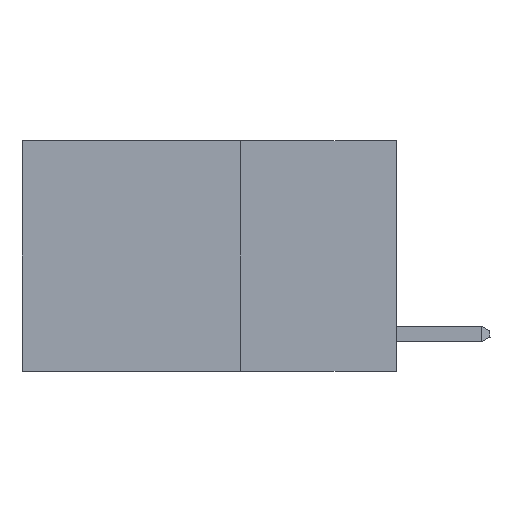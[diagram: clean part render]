
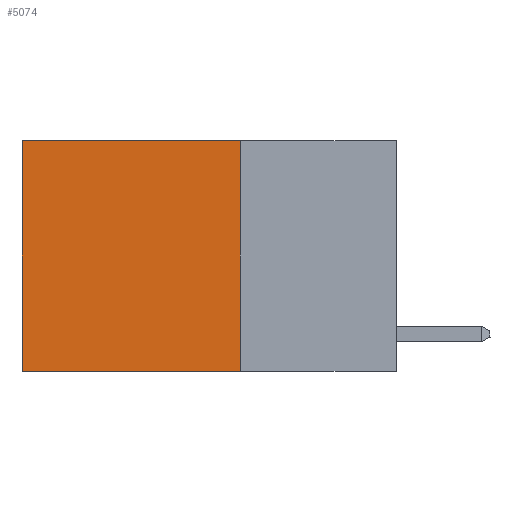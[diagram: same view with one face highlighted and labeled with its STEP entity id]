
A CAD part, left-side view. The second image highlights one B-rep face of the part: STEP entity #5074.
In plain terms, the highlighted planar face has unit normal (-1, 0, 0).
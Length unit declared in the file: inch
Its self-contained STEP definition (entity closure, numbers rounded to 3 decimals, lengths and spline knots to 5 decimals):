
#591 = LINE ( 'NONE', #10597, #12261 ) ;
#614 = VECTOR ( 'NONE', #5404, 39.37008 ) ;
#617 = CARTESIAN_POINT ( 'NONE',  ( 0.2625, 0.25, 0. ) ) ;
#834 = ORIENTED_EDGE ( 'NONE', *, *, #8151, .F. ) ;
#877 = CARTESIAN_POINT ( 'NONE',  ( 0.2625, 0.25, 0. ) ) ;
#1131 = DIRECTION ( 'NONE',  ( 0., 0., -1. ) ) ;
#1526 = VERTEX_POINT ( 'NONE', #4899 ) ;
#1620 = CARTESIAN_POINT ( 'NONE',  ( 0.2625, 0.6, 0. ) ) ;
#3361 = CARTESIAN_POINT ( 'NONE',  ( 0.2625, 0.25, 0. ) ) ;
#3754 = CARTESIAN_POINT ( 'NONE',  ( 0.2625, 0.6, -0.37 ) ) ;
#3759 = ORIENTED_EDGE ( 'NONE', *, *, #8839, .T. ) ;
#3960 = LINE ( 'NONE', #8099, #12637 ) ;
#4899 = CARTESIAN_POINT ( 'NONE',  ( 0.2625, 0.25, -0.37 ) ) ;
#5074 = ADVANCED_FACE ( 'NONE', ( #6721 ), #5600, .F. ) ;
#5404 = DIRECTION ( 'NONE',  ( 0., 1., 0. ) ) ;
#5600 = PLANE ( 'NONE',  #6029 ) ;
#6029 = AXIS2_PLACEMENT_3D ( 'NONE', #3361, #7900, #1131 ) ;
#6721 = FACE_OUTER_BOUND ( 'NONE', #7331, .T. ) ;
#7331 = EDGE_LOOP ( 'NONE', ( #3759, #9651, #834, #7700 ) ) ;
#7636 = DIRECTION ( 'NONE',  ( 0., 0., -1. ) ) ;
#7700 = ORIENTED_EDGE ( 'NONE', *, *, #9796, .T. ) ;
#7900 = DIRECTION ( 'NONE',  ( 1., 0., 0. ) ) ;
#8099 = CARTESIAN_POINT ( 'NONE',  ( 0.2625, 0.6, 0. ) ) ;
#8151 = EDGE_CURVE ( 'NONE', #13231, #1526, #8583, .T. ) ;
#8583 = LINE ( 'NONE', #877, #14257 ) ;
#8839 = EDGE_CURVE ( 'NONE', #14494, #13821, #3960, .T. ) ;
#9264 = DIRECTION ( 'NONE',  ( 0., 0., -1. ) ) ;
#9275 = LINE ( 'NONE', #12210, #614 ) ;
#9651 = ORIENTED_EDGE ( 'NONE', *, *, #14117, .F. ) ;
#9796 = EDGE_CURVE ( 'NONE', #13231, #14494, #591, .T. ) ;
#10597 = CARTESIAN_POINT ( 'NONE',  ( 0.2625, 0.25, 0. ) ) ;
#12210 = CARTESIAN_POINT ( 'NONE',  ( 0.2625, 0.25, -0.37 ) ) ;
#12261 = VECTOR ( 'NONE', #12796, 39.37008 ) ;
#12637 = VECTOR ( 'NONE', #9264, 39.37008 ) ;
#12796 = DIRECTION ( 'NONE',  ( 0., 1., 0. ) ) ;
#13231 = VERTEX_POINT ( 'NONE', #617 ) ;
#13821 = VERTEX_POINT ( 'NONE', #3754 ) ;
#14117 = EDGE_CURVE ( 'NONE', #1526, #13821, #9275, .T. ) ;
#14257 = VECTOR ( 'NONE', #7636, 39.37008 ) ;
#14494 = VERTEX_POINT ( 'NONE', #1620 ) ;
